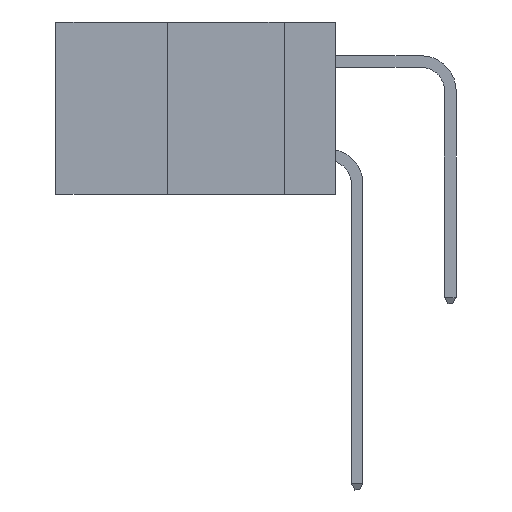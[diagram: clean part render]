
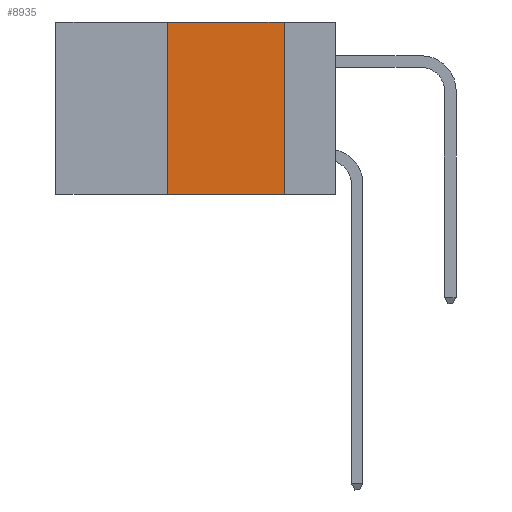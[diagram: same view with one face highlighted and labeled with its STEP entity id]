
A CAD part, left-side view. The second image highlights one B-rep face of the part: STEP entity #8935.
In plain terms, the highlighted planar face has unit normal (-1, 0, 0).
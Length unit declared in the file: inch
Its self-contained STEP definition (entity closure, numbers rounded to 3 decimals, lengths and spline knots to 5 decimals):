
#392 = CARTESIAN_POINT ( 'NONE',  ( 0., 0.6, 0. ) ) ;
#505 = VECTOR ( 'NONE', #4461, 39.37008 ) ;
#591 = LINE ( 'NONE', #12771, #6497 ) ;
#962 = VERTEX_POINT ( 'NONE', #13228 ) ;
#1187 = EDGE_CURVE ( 'NONE', #13396, #9850, #8277, .T. ) ;
#1292 = EDGE_CURVE ( 'NONE', #9850, #11807, #6796, .T. ) ;
#1447 = CARTESIAN_POINT ( 'NONE',  ( 0., 0.11, -0.37 ) ) ;
#1637 = PLANE ( 'NONE',  #14567 ) ;
#1858 = ORIENTED_EDGE ( 'NONE', *, *, #1187, .F. ) ;
#2611 = FACE_OUTER_BOUND ( 'NONE', #4230, .T. ) ;
#2806 = DIRECTION ( 'NONE',  ( 1., 0., 0. ) ) ;
#3529 = CARTESIAN_POINT ( 'NONE',  ( 0., 0.11, 0. ) ) ;
#3835 = CARTESIAN_POINT ( 'NONE',  ( 0., 0.36, 0. ) ) ;
#3937 = CARTESIAN_POINT ( 'NONE',  ( 0., 0.11, 0. ) ) ;
#4089 = VECTOR ( 'NONE', #8251, 39.37008 ) ;
#4230 = EDGE_LOOP ( 'NONE', ( #10292, #1858, #5885, #13298 ) ) ;
#4364 = VECTOR ( 'NONE', #11193, 39.37008 ) ;
#4461 = DIRECTION ( 'NONE',  ( 0., 0., -1. ) ) ;
#4632 = CARTESIAN_POINT ( 'NONE',  ( 0., 0.36, 0. ) ) ;
#5085 = CARTESIAN_POINT ( 'NONE',  ( 0., 0.6, 0. ) ) ;
#5885 = ORIENTED_EDGE ( 'NONE', *, *, #9151, .F. ) ;
#6497 = VECTOR ( 'NONE', #9634, 39.37008 ) ;
#6796 = LINE ( 'NONE', #3937, #505 ) ;
#8251 = DIRECTION ( 'NONE',  ( 0., 0., 1. ) ) ;
#8277 = LINE ( 'NONE', #392, #4364 ) ;
#8935 = ADVANCED_FACE ( 'NONE', ( #2611 ), #1637, .F. ) ;
#9151 = EDGE_CURVE ( 'NONE', #962, #13396, #12972, .T. ) ;
#9634 = DIRECTION ( 'NONE',  ( 0., -1., 0. ) ) ;
#9850 = VERTEX_POINT ( 'NONE', #3529 ) ;
#10292 = ORIENTED_EDGE ( 'NONE', *, *, #1292, .F. ) ;
#10762 = DIRECTION ( 'NONE',  ( 0., 0., -1. ) ) ;
#11193 = DIRECTION ( 'NONE',  ( 0., -1., 0. ) ) ;
#11807 = VERTEX_POINT ( 'NONE', #1447 ) ;
#12771 = CARTESIAN_POINT ( 'NONE',  ( 0., 0.6, -0.37 ) ) ;
#12972 = LINE ( 'NONE', #4632, #4089 ) ;
#13228 = CARTESIAN_POINT ( 'NONE',  ( 0., 0.36, -0.37 ) ) ;
#13298 = ORIENTED_EDGE ( 'NONE', *, *, #13413, .T. ) ;
#13396 = VERTEX_POINT ( 'NONE', #3835 ) ;
#13413 = EDGE_CURVE ( 'NONE', #962, #11807, #591, .T. ) ;
#14567 = AXIS2_PLACEMENT_3D ( 'NONE', #5085, #2806, #10762 ) ;
